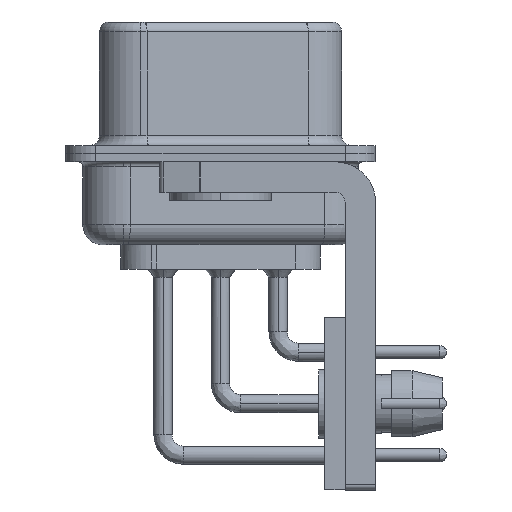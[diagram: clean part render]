
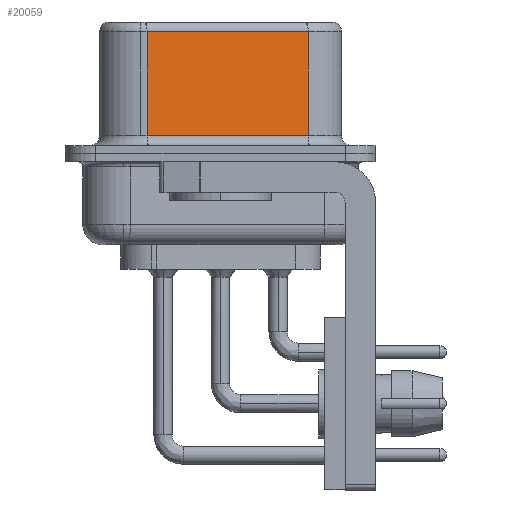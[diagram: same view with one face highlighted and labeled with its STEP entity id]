
A CAD part, left-side view. The second image highlights one B-rep face of the part: STEP entity #20059.
In plain terms, the highlighted planar face has unit normal (-0.985, -0.174, 0).
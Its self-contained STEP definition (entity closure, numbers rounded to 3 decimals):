
#5 = CARTESIAN_POINT ( 'NONE',  ( 5.132, -4.322, 0.9 ) ) ;
#889 = CARTESIAN_POINT ( 'NONE',  ( 3.73, 3.628, 6.02 ) ) ;
#925 = DIRECTION ( 'NONE',  ( 0.985, 0.174, 0. ) ) ;
#1403 = LINE ( 'NONE', #29913, #35118 ) ;
#2149 = ORIENTED_EDGE ( 'NONE', *, *, #13306, .T. ) ;
#3603 = EDGE_CURVE ( 'NONE', #32770, #31060, #1403, .T. ) ;
#3972 = VERTEX_POINT ( 'NONE', #38159 ) ;
#4291 = CARTESIAN_POINT ( 'NONE',  ( 5.132, -4.322, 6.52 ) ) ;
#4820 = FACE_OUTER_BOUND ( 'NONE', #41585, .T. ) ;
#6341 = LINE ( 'NONE', #9903, #40079 ) ;
#7474 = EDGE_CURVE ( 'NONE', #16980, #32770, #6341, .T. ) ;
#9903 = CARTESIAN_POINT ( 'NONE',  ( 3.73, 3.628, 6.52 ) ) ;
#11060 = DIRECTION ( 'NONE',  ( -0.174, 0.985, 0. ) ) ;
#11932 = LINE ( 'NONE', #32287, #18705 ) ;
#12552 = AXIS2_PLACEMENT_3D ( 'NONE', #4291, #925, #11060 ) ;
#13306 = EDGE_CURVE ( 'NONE', #3972, #16980, #11932, .T. ) ;
#16147 = VECTOR ( 'NONE', #16684, 1000. ) ;
#16331 = EDGE_CURVE ( 'NONE', #3972, #31060, #25054, .T. ) ;
#16684 = DIRECTION ( 'NONE',  ( 0., 0., -1. ) ) ;
#16980 = VERTEX_POINT ( 'NONE', #889 ) ;
#18372 = ORIENTED_EDGE ( 'NONE', *, *, #7474, .T. ) ;
#18705 = VECTOR ( 'NONE', #22075, 1000. ) ;
#20059 = ADVANCED_FACE ( 'NONE', ( #4820 ), #31205, .F. ) ;
#20679 = ORIENTED_EDGE ( 'NONE', *, *, #3603, .T. ) ;
#22075 = DIRECTION ( 'NONE',  ( -0.174, 0.985, 0. ) ) ;
#23955 = CARTESIAN_POINT ( 'NONE',  ( 3.73, 3.628, 0.9 ) ) ;
#25054 = LINE ( 'NONE', #36943, #16147 ) ;
#29913 = CARTESIAN_POINT ( 'NONE',  ( 5.132, -4.322, 0.9 ) ) ;
#30647 = DIRECTION ( 'NONE',  ( 0.174, -0.985, 0. ) ) ;
#31060 = VERTEX_POINT ( 'NONE', #5 ) ;
#31205 = PLANE ( 'NONE',  #12552 ) ;
#32287 = CARTESIAN_POINT ( 'NONE',  ( 5.132, -4.322, 6.02 ) ) ;
#32770 = VERTEX_POINT ( 'NONE', #23955 ) ;
#33457 = DIRECTION ( 'NONE',  ( 0., 0., -1. ) ) ;
#35118 = VECTOR ( 'NONE', #30647, 1000. ) ;
#36943 = CARTESIAN_POINT ( 'NONE',  ( 5.132, -4.322, 6.52 ) ) ;
#38159 = CARTESIAN_POINT ( 'NONE',  ( 5.132, -4.322, 6.02 ) ) ;
#40079 = VECTOR ( 'NONE', #33457, 1000. ) ;
#41585 = EDGE_LOOP ( 'NONE', ( #43664, #2149, #18372, #20679 ) ) ;
#43664 = ORIENTED_EDGE ( 'NONE', *, *, #16331, .F. ) ;
